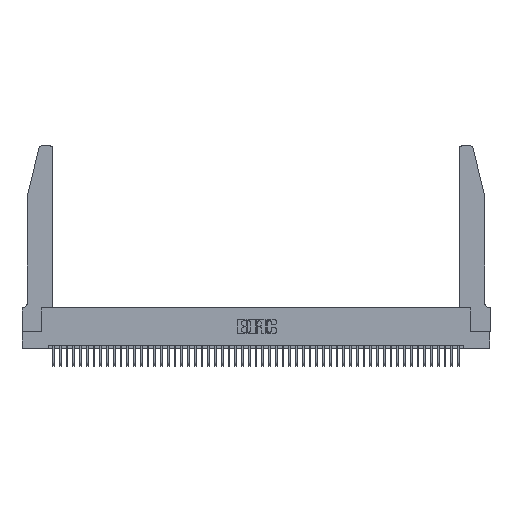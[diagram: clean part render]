
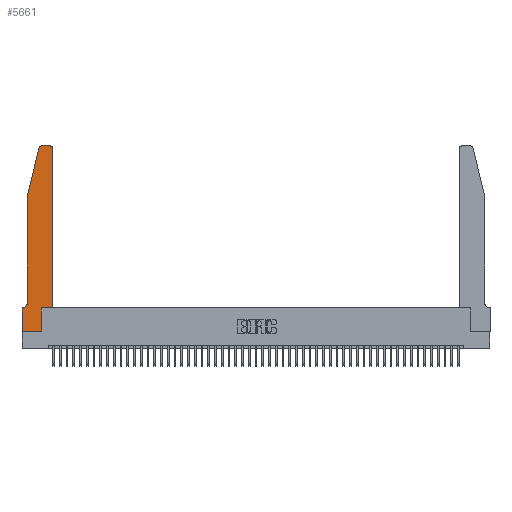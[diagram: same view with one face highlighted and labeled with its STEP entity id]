
A CAD part, top view. The second image highlights one B-rep face of the part: STEP entity #5661.
In plain terms, the highlighted planar face has unit normal (0, 0, 1).
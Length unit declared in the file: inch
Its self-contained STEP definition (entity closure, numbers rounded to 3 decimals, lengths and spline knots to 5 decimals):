
#29 = EDGE_CURVE ( 'NONE', #28505, #47493, #19502, .T. ) ;
#106 = DIRECTION ( 'NONE',  ( 0., 1., 0. ) ) ;
#597 = CARTESIAN_POINT ( 'NONE',  ( 0.2605, 2.75, 0.37 ) ) ;
#898 = CARTESIAN_POINT ( 'NONE',  ( 0.4505, 2.72, 0.37 ) ) ;
#973 = PLANE ( 'NONE',  #42742 ) ;
#1135 = VERTEX_POINT ( 'NONE', #29876 ) ;
#1384 = EDGE_CURVE ( 'NONE', #8235, #41175, #38073, .T. ) ;
#1444 = CARTESIAN_POINT ( 'NONE',  ( 0.25487, 2.72718, 0.37 ) ) ;
#2192 = ORIENTED_EDGE ( 'NONE', *, *, #26193, .T. ) ;
#3524 = CARTESIAN_POINT ( 'NONE',  ( 0.4505, 0.35, 0.37 ) ) ;
#3756 = EDGE_CURVE ( 'NONE', #10990, #1135, #22631, .T. ) ;
#4639 = VERTEX_POINT ( 'NONE', #6450 ) ;
#5253 = CARTESIAN_POINT ( 'NONE',  ( 0.2865, 0.35, 0.37 ) ) ;
#5629 = DIRECTION ( 'NONE',  ( -0.239, -0.971, 0. ) ) ;
#5661 = ADVANCED_FACE ( 'NONE', ( #24173 ), #973, .T. ) ;
#6051 = LINE ( 'NONE', #31670, #43922 ) ;
#6142 = VERTEX_POINT ( 'NONE', #37605 ) ;
#6257 = CARTESIAN_POINT ( 'NONE',  ( 0.0055, 0.42, 0.37 ) ) ;
#6450 = CARTESIAN_POINT ( 'NONE',  ( 0.4505, 0.35, 0.37 ) ) ;
#6587 = CIRCLE ( 'NONE', #26200, 0.03 ) ;
#7281 = DIRECTION ( 'NONE',  ( 1., 0., 0. ) ) ;
#8235 = VERTEX_POINT ( 'NONE', #22596 ) ;
#8856 = DIRECTION ( 'NONE',  ( 0., -1., 0. ) ) ;
#9098 = EDGE_CURVE ( 'NONE', #46484, #23642, #20183, .T. ) ;
#9227 = CARTESIAN_POINT ( 'NONE',  ( 0., 0., 0.37 ) ) ;
#9791 = VECTOR ( 'NONE', #43422, 39.37008 ) ;
#9990 = DIRECTION ( 'NONE',  ( -1., 0., 0. ) ) ;
#10068 = ORIENTED_EDGE ( 'NONE', *, *, #18421, .T. ) ;
#10309 = VECTOR ( 'NONE', #24482, 39.37008 ) ;
#10591 = VECTOR ( 'NONE', #30401, 39.37008 ) ;
#10990 = VERTEX_POINT ( 'NONE', #898 ) ;
#11246 = CARTESIAN_POINT ( 'NONE',  ( 0.0755, 0.35, 0.37 ) ) ;
#11285 = ORIENTED_EDGE ( 'NONE', *, *, #45915, .T. ) ;
#12044 = DIRECTION ( 'NONE',  ( 0., 0., 1. ) ) ;
#13719 = EDGE_CURVE ( 'NONE', #41175, #6142, #31395, .T. ) ;
#13931 = VECTOR ( 'NONE', #28215, 39.37008 ) ;
#14882 = CARTESIAN_POINT ( 'NONE',  ( 0., 0.35, 0.37 ) ) ;
#15109 = LINE ( 'NONE', #24462, #13931 ) ;
#15930 = CARTESIAN_POINT ( 'NONE',  ( 0., 0.35, 0.37 ) ) ;
#16630 = EDGE_CURVE ( 'NONE', #1135, #40714, #40310, .T. ) ;
#17172 = CARTESIAN_POINT ( 'NONE',  ( 0., 0., 0.37 ) ) ;
#17273 = DIRECTION ( 'NONE',  ( 0., 0., 1. ) ) ;
#17939 = ORIENTED_EDGE ( 'NONE', *, *, #3756, .T. ) ;
#17962 = VECTOR ( 'NONE', #7281, 39.37008 ) ;
#18421 = EDGE_CURVE ( 'NONE', #47493, #4639, #47627, .T. ) ;
#18598 = ORIENTED_EDGE ( 'NONE', *, *, #33625, .T. ) ;
#19502 = LINE ( 'NONE', #5253, #38209 ) ;
#19667 = DIRECTION ( 'NONE',  ( 1., 0., 0. ) ) ;
#19880 = ORIENTED_EDGE ( 'NONE', *, *, #29, .T. ) ;
#19913 = AXIS2_PLACEMENT_3D ( 'NONE', #34397, #12044, #38121 ) ;
#20183 = LINE ( 'NONE', #17172, #10309 ) ;
#20765 = CARTESIAN_POINT ( 'NONE',  ( 0.2865, 0.35, 0.37 ) ) ;
#20845 = ORIENTED_EDGE ( 'NONE', *, *, #1384, .T. ) ;
#21122 = CARTESIAN_POINT ( 'NONE',  ( 0., 0., 0.37 ) ) ;
#21130 = CARTESIAN_POINT ( 'NONE',  ( 0.2865, 0., 0.37 ) ) ;
#21811 = EDGE_CURVE ( 'NONE', #4639, #10990, #15109, .T. ) ;
#22596 = CARTESIAN_POINT ( 'NONE',  ( 0.0755, 2., 0.37 ) ) ;
#22631 = CIRCLE ( 'NONE', #19913, 0.03 ) ;
#23613 = CARTESIAN_POINT ( 'NONE',  ( 0.284, 2.75, 0.37 ) ) ;
#23642 = VERTEX_POINT ( 'NONE', #9227 ) ;
#24173 = FACE_OUTER_BOUND ( 'NONE', #41488, .T. ) ;
#24462 = CARTESIAN_POINT ( 'NONE',  ( 0.4505, 0.35, 0.37 ) ) ;
#24482 = DIRECTION ( 'NONE',  ( 0., -1., 0. ) ) ;
#26193 = EDGE_CURVE ( 'NONE', #40714, #47403, #6587, .T. ) ;
#26200 = AXIS2_PLACEMENT_3D ( 'NONE', #39607, #17273, #43298 ) ;
#26211 = CARTESIAN_POINT ( 'NONE',  ( 0.0755, 0.42, 0.37 ) ) ;
#27820 = ORIENTED_EDGE ( 'NONE', *, *, #37814, .T. ) ;
#28089 = VECTOR ( 'NONE', #8856, 39.37008 ) ;
#28215 = DIRECTION ( 'NONE',  ( 0., 1., 0. ) ) ;
#28505 = VERTEX_POINT ( 'NONE', #21130 ) ;
#29876 = CARTESIAN_POINT ( 'NONE',  ( 0.4205, 2.75, 0.37 ) ) ;
#30401 = DIRECTION ( 'NONE',  ( -1., 0., 0. ) ) ;
#31395 = CIRCLE ( 'NONE', #32056, 0.07 ) ;
#31670 = CARTESIAN_POINT ( 'NONE',  ( 0.0755, 2., 0.37 ) ) ;
#32056 = AXIS2_PLACEMENT_3D ( 'NONE', #6257, #32314, #9990 ) ;
#32314 = DIRECTION ( 'NONE',  ( 0., 0., -1. ) ) ;
#33231 = ORIENTED_EDGE ( 'NONE', *, *, #16630, .T. ) ;
#33305 = ORIENTED_EDGE ( 'NONE', *, *, #21811, .T. ) ;
#33625 = EDGE_CURVE ( 'NONE', #23642, #28505, #39514, .T. ) ;
#34397 = CARTESIAN_POINT ( 'NONE',  ( 0.4205, 2.72, 0.37 ) ) ;
#36860 = VECTOR ( 'NONE', #41032, 39.37008 ) ;
#37605 = CARTESIAN_POINT ( 'NONE',  ( 0.0055, 0.35, 0.37 ) ) ;
#37814 = EDGE_CURVE ( 'NONE', #6142, #46484, #47814, .T. ) ;
#38073 = LINE ( 'NONE', #38665, #28089 ) ;
#38121 = DIRECTION ( 'NONE',  ( 1., 0., 0. ) ) ;
#38209 = VECTOR ( 'NONE', #106, 39.37008 ) ;
#38665 = CARTESIAN_POINT ( 'NONE',  ( 0.0755, 2., 0.37 ) ) ;
#39514 = LINE ( 'NONE', #21122, #9791 ) ;
#39607 = CARTESIAN_POINT ( 'NONE',  ( 0.284, 2.72, 0.37 ) ) ;
#40310 = LINE ( 'NONE', #597, #10591 ) ;
#40714 = VERTEX_POINT ( 'NONE', #23613 ) ;
#41032 = DIRECTION ( 'NONE',  ( -1., 0., 0. ) ) ;
#41175 = VERTEX_POINT ( 'NONE', #26211 ) ;
#41488 = EDGE_LOOP ( 'NONE', ( #33231, #2192, #11285, #20845, #42337, #27820, #42681, #18598, #19880, #10068, #33305, #17939 ) ) ;
#41976 = DIRECTION ( 'NONE',  ( 0., 0., 1. ) ) ;
#42337 = ORIENTED_EDGE ( 'NONE', *, *, #13719, .T. ) ;
#42681 = ORIENTED_EDGE ( 'NONE', *, *, #9098, .T. ) ;
#42742 = AXIS2_PLACEMENT_3D ( 'NONE', #15930, #41976, #19667 ) ;
#43298 = DIRECTION ( 'NONE',  ( 1., 0., 0. ) ) ;
#43422 = DIRECTION ( 'NONE',  ( 1., 0., 0. ) ) ;
#43922 = VECTOR ( 'NONE', #5629, 39.37008 ) ;
#45915 = EDGE_CURVE ( 'NONE', #47403, #8235, #6051, .T. ) ;
#46484 = VERTEX_POINT ( 'NONE', #14882 ) ;
#47403 = VERTEX_POINT ( 'NONE', #1444 ) ;
#47493 = VERTEX_POINT ( 'NONE', #20765 ) ;
#47627 = LINE ( 'NONE', #3524, #17962 ) ;
#47814 = LINE ( 'NONE', #11246, #36860 ) ;
